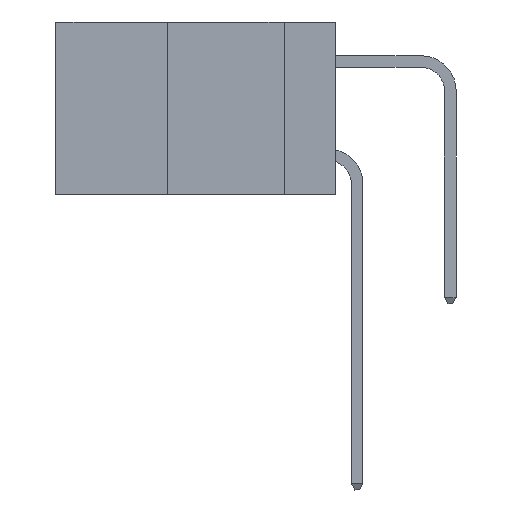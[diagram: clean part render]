
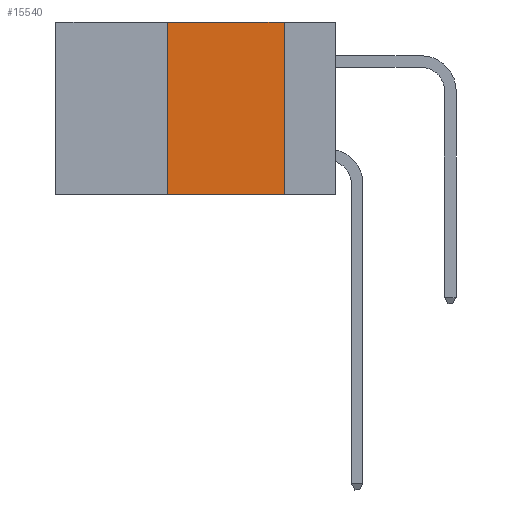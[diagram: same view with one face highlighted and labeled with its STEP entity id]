
A CAD part, left-side view. The second image highlights one B-rep face of the part: STEP entity #15540.
In plain terms, the highlighted planar face has unit normal (-1, 0, 0).
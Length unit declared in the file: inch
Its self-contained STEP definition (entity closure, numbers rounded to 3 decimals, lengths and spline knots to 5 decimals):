
#686 = ORIENTED_EDGE ( 'NONE', *, *, #5711, .F. ) ;
#1715 = VERTEX_POINT ( 'NONE', #18025 ) ;
#1935 = EDGE_CURVE ( 'NONE', #23521, #19587, #19106, .T. ) ;
#2475 = LINE ( 'NONE', #14240, #17940 ) ;
#3232 = EDGE_LOOP ( 'NONE', ( #686, #17164, #19834, #22526 ) ) ;
#4458 = EDGE_CURVE ( 'NONE', #1715, #6539, #21166, .T. ) ;
#5711 = EDGE_CURVE ( 'NONE', #19587, #6539, #2475, .T. ) ;
#6378 = CARTESIAN_POINT ( 'NONE',  ( 0., 0.36, 0. ) ) ;
#6539 = VERTEX_POINT ( 'NONE', #22915 ) ;
#6921 = CARTESIAN_POINT ( 'NONE',  ( 0., 0.36, 0. ) ) ;
#10596 = VECTOR ( 'NONE', #27392, 39.37008 ) ;
#11926 = CARTESIAN_POINT ( 'NONE',  ( 0., 0.6, -0.37 ) ) ;
#11931 = CARTESIAN_POINT ( 'NONE',  ( 0., 0.6, 0. ) ) ;
#14240 = CARTESIAN_POINT ( 'NONE',  ( 0., 0.11, 0. ) ) ;
#15146 = AXIS2_PLACEMENT_3D ( 'NONE', #11931, #34855, #17834 ) ;
#15355 = VECTOR ( 'NONE', #31889, 39.37008 ) ;
#15540 = ADVANCED_FACE ( 'NONE', ( #23275 ), #26348, .F. ) ;
#17164 = ORIENTED_EDGE ( 'NONE', *, *, #1935, .F. ) ;
#17834 = DIRECTION ( 'NONE',  ( 0., 0., -1. ) ) ;
#17940 = VECTOR ( 'NONE', #31308, 39.37008 ) ;
#18025 = CARTESIAN_POINT ( 'NONE',  ( 0., 0.36, -0.37 ) ) ;
#18874 = CARTESIAN_POINT ( 'NONE',  ( 0., 0.6, 0. ) ) ;
#19106 = LINE ( 'NONE', #18874, #10596 ) ;
#19587 = VERTEX_POINT ( 'NONE', #22055 ) ;
#19834 = ORIENTED_EDGE ( 'NONE', *, *, #29486, .F. ) ;
#21166 = LINE ( 'NONE', #11926, #15355 ) ;
#21788 = VECTOR ( 'NONE', #24110, 39.37008 ) ;
#22055 = CARTESIAN_POINT ( 'NONE',  ( 0., 0.11, 0. ) ) ;
#22526 = ORIENTED_EDGE ( 'NONE', *, *, #4458, .T. ) ;
#22915 = CARTESIAN_POINT ( 'NONE',  ( 0., 0.11, -0.37 ) ) ;
#23275 = FACE_OUTER_BOUND ( 'NONE', #3232, .T. ) ;
#23521 = VERTEX_POINT ( 'NONE', #6378 ) ;
#24110 = DIRECTION ( 'NONE',  ( 0., 0., 1. ) ) ;
#26348 = PLANE ( 'NONE',  #15146 ) ;
#27392 = DIRECTION ( 'NONE',  ( 0., -1., 0. ) ) ;
#29361 = LINE ( 'NONE', #6921, #21788 ) ;
#29486 = EDGE_CURVE ( 'NONE', #1715, #23521, #29361, .T. ) ;
#31308 = DIRECTION ( 'NONE',  ( 0., 0., -1. ) ) ;
#31889 = DIRECTION ( 'NONE',  ( 0., -1., 0. ) ) ;
#34855 = DIRECTION ( 'NONE',  ( 1., 0., 0. ) ) ;
